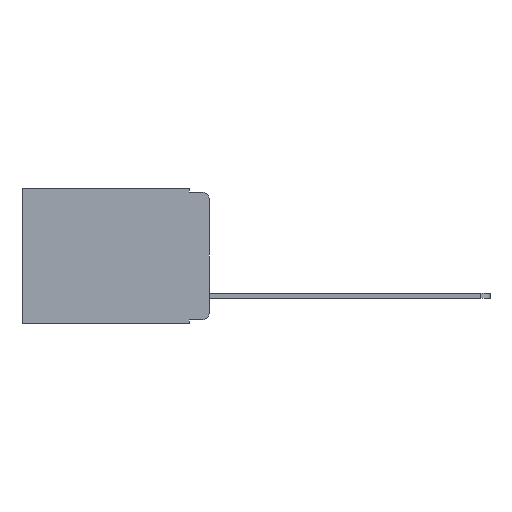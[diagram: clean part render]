
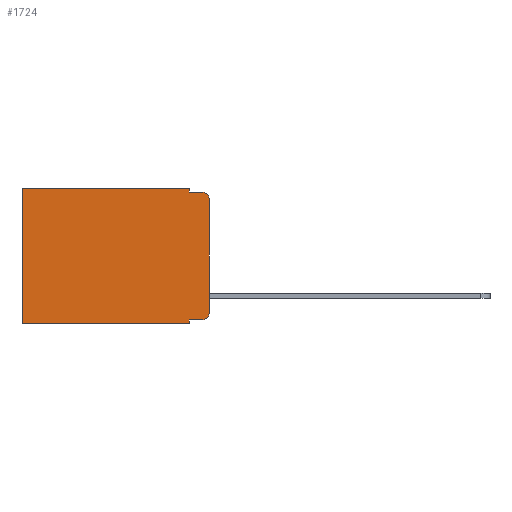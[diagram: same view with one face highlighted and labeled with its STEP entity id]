
A CAD part, left-side view. The second image highlights one B-rep face of the part: STEP entity #1724.
In plain terms, the highlighted planar face has unit normal (-1, 0, 0).
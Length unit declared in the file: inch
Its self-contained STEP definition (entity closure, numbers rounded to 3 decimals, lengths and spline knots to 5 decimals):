
#91 = ORIENTED_EDGE ( 'NONE', *, *, #9398, .F. ) ;
#135 = VECTOR ( 'NONE', #3371, 39.37008 ) ;
#203 = CARTESIAN_POINT ( 'NONE',  ( 0.298, 0.02, -0.313 ) ) ;
#230 = AXIS2_PLACEMENT_3D ( 'NONE', #4660, #5311, #3256 ) ;
#510 = VERTEX_POINT ( 'NONE', #5341 ) ;
#584 = LINE ( 'NONE', #9635, #6694 ) ;
#686 = ORIENTED_EDGE ( 'NONE', *, *, #7618, .F. ) ;
#839 = DIRECTION ( 'NONE',  ( -1., 0., 0. ) ) ;
#966 = CIRCLE ( 'NONE', #4983, 0.02 ) ;
#983 = ORIENTED_EDGE ( 'NONE', *, *, #1739, .T. ) ;
#1027 = CARTESIAN_POINT ( 'NONE',  ( 0.298, 0., -0.343 ) ) ;
#1093 = DIRECTION ( 'NONE',  ( 0., 0., -1. ) ) ;
#1197 = ORIENTED_EDGE ( 'NONE', *, *, #4644, .F. ) ;
#1387 = ORIENTED_EDGE ( 'NONE', *, *, #9199, .T. ) ;
#1388 = CARTESIAN_POINT ( 'NONE',  ( 0.298, 0., 0. ) ) ;
#1477 = CARTESIAN_POINT ( 'NONE',  ( 0.298, 0.051, -0.333 ) ) ;
#1674 = EDGE_CURVE ( 'NONE', #6648, #3746, #3395, .T. ) ;
#1724 = ADVANCED_FACE ( 'NONE', ( #8408 ), #5469, .F. ) ;
#1739 = EDGE_CURVE ( 'NONE', #3746, #4046, #6582, .T. ) ;
#1854 = ORIENTED_EDGE ( 'NONE', *, *, #2286, .F. ) ;
#1891 = LINE ( 'NONE', #5930, #5868 ) ;
#2070 = VERTEX_POINT ( 'NONE', #6857 ) ;
#2286 = EDGE_CURVE ( 'NONE', #2070, #4046, #9755, .T. ) ;
#2290 = EDGE_CURVE ( 'NONE', #6840, #2070, #1891, .T. ) ;
#2810 = CARTESIAN_POINT ( 'NONE',  ( 0.298, 0.051, -0.333 ) ) ;
#3028 = CARTESIAN_POINT ( 'NONE',  ( 0.298, 0.051, -0.01 ) ) ;
#3256 = DIRECTION ( 'NONE',  ( 0., 0., -1. ) ) ;
#3371 = DIRECTION ( 'NONE',  ( 0., 0., -1. ) ) ;
#3395 = LINE ( 'NONE', #1388, #7016 ) ;
#3464 = VERTEX_POINT ( 'NONE', #7885 ) ;
#3574 = VERTEX_POINT ( 'NONE', #6292 ) ;
#3746 = VERTEX_POINT ( 'NONE', #4500 ) ;
#4004 = LINE ( 'NONE', #7972, #6067 ) ;
#4006 = ORIENTED_EDGE ( 'NONE', *, *, #7143, .T. ) ;
#4046 = VERTEX_POINT ( 'NONE', #8335 ) ;
#4123 = CARTESIAN_POINT ( 'NONE',  ( 0.298, 0.051, 0. ) ) ;
#4302 = EDGE_LOOP ( 'NONE', ( #1197, #4006, #686, #91, #6412, #983, #1854, #6010, #7879, #1387 ) ) ;
#4500 = CARTESIAN_POINT ( 'NONE',  ( 0.298, 0.473, 0. ) ) ;
#4590 = CARTESIAN_POINT ( 'NONE',  ( 0.298, 0.051, 0. ) ) ;
#4644 = EDGE_CURVE ( 'NONE', #6895, #3464, #4004, .T. ) ;
#4660 = CARTESIAN_POINT ( 'NONE',  ( 0.298, 0., 0. ) ) ;
#4694 = DIRECTION ( 'NONE',  ( 0., -1., 0. ) ) ;
#4975 = EDGE_CURVE ( 'NONE', #6840, #3574, #5212, .T. ) ;
#4983 = AXIS2_PLACEMENT_3D ( 'NONE', #203, #5903, #1093 ) ;
#4986 = VECTOR ( 'NONE', #5820, 39.37008 ) ;
#5094 = VERTEX_POINT ( 'NONE', #3028 ) ;
#5212 = LINE ( 'NONE', #1477, #4986 ) ;
#5311 = DIRECTION ( 'NONE',  ( 1., 0., 0. ) ) ;
#5341 = CARTESIAN_POINT ( 'NONE',  ( 0.298, 0.02, -0.01 ) ) ;
#5469 = PLANE ( 'NONE',  #230 ) ;
#5682 = CARTESIAN_POINT ( 'NONE',  ( 0.298, 0.02, -0.03 ) ) ;
#5820 = DIRECTION ( 'NONE',  ( 0., -1., 0. ) ) ;
#5868 = VECTOR ( 'NONE', #6063, 39.37008 ) ;
#5903 = DIRECTION ( 'NONE',  ( -1., 0., 0. ) ) ;
#5930 = CARTESIAN_POINT ( 'NONE',  ( 0.298, 0.051, 0. ) ) ;
#6010 = ORIENTED_EDGE ( 'NONE', *, *, #2290, .F. ) ;
#6063 = DIRECTION ( 'NONE',  ( 0., 0., -1. ) ) ;
#6067 = VECTOR ( 'NONE', #8883, 39.37008 ) ;
#6292 = CARTESIAN_POINT ( 'NONE',  ( 0.298, 0.02, -0.333 ) ) ;
#6412 = ORIENTED_EDGE ( 'NONE', *, *, #1674, .T. ) ;
#6435 = DIRECTION ( 'NONE',  ( 0., 0., -1. ) ) ;
#6582 = LINE ( 'NONE', #9815, #135 ) ;
#6648 = VERTEX_POINT ( 'NONE', #4123 ) ;
#6694 = VECTOR ( 'NONE', #4694, 39.37008 ) ;
#6773 = CARTESIAN_POINT ( 'NONE',  ( 0.298, 0., -0.03 ) ) ;
#6824 = DIRECTION ( 'NONE',  ( 0., 0., -1. ) ) ;
#6840 = VERTEX_POINT ( 'NONE', #2810 ) ;
#6857 = CARTESIAN_POINT ( 'NONE',  ( 0.298, 0.051, -0.343 ) ) ;
#6895 = VERTEX_POINT ( 'NONE', #6773 ) ;
#7016 = VECTOR ( 'NONE', #8007, 39.37008 ) ;
#7143 = EDGE_CURVE ( 'NONE', #6895, #510, #9167, .T. ) ;
#7324 = VECTOR ( 'NONE', #6824, 39.37008 ) ;
#7618 = EDGE_CURVE ( 'NONE', #5094, #510, #584, .T. ) ;
#7879 = ORIENTED_EDGE ( 'NONE', *, *, #4975, .T. ) ;
#7885 = CARTESIAN_POINT ( 'NONE',  ( 0.298, 0., -0.313 ) ) ;
#7972 = CARTESIAN_POINT ( 'NONE',  ( 0.298, 0., 0. ) ) ;
#8007 = DIRECTION ( 'NONE',  ( 0., 1., 0. ) ) ;
#8335 = CARTESIAN_POINT ( 'NONE',  ( 0.298, 0.473, -0.343 ) ) ;
#8408 = FACE_OUTER_BOUND ( 'NONE', #4302, .T. ) ;
#8430 = DIRECTION ( 'NONE',  ( 0., 1., 0. ) ) ;
#8498 = LINE ( 'NONE', #4590, #7324 ) ;
#8883 = DIRECTION ( 'NONE',  ( 0., 0., -1. ) ) ;
#9167 = CIRCLE ( 'NONE', #9734, 0.02 ) ;
#9199 = EDGE_CURVE ( 'NONE', #3574, #3464, #966, .T. ) ;
#9398 = EDGE_CURVE ( 'NONE', #6648, #5094, #8498, .T. ) ;
#9538 = VECTOR ( 'NONE', #8430, 39.37008 ) ;
#9635 = CARTESIAN_POINT ( 'NONE',  ( 0.298, 0.051, -0.01 ) ) ;
#9734 = AXIS2_PLACEMENT_3D ( 'NONE', #5682, #839, #6435 ) ;
#9755 = LINE ( 'NONE', #1027, #9538 ) ;
#9815 = CARTESIAN_POINT ( 'NONE',  ( 0.298, 0.473, 0. ) ) ;
